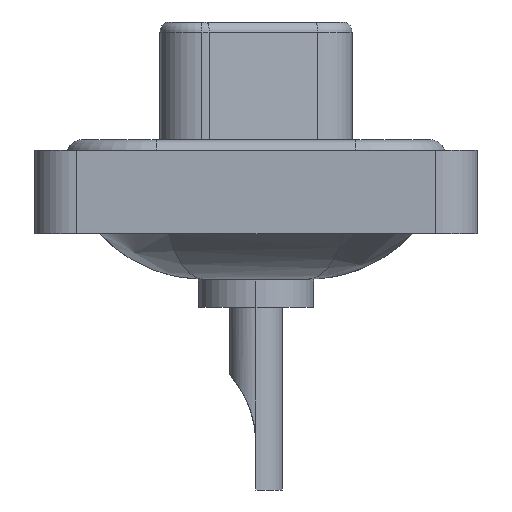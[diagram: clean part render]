
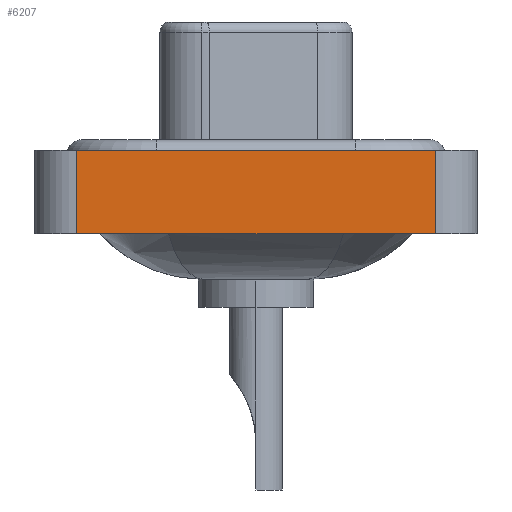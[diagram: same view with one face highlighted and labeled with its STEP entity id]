
A CAD part, left-side view. The second image highlights one B-rep face of the part: STEP entity #6207.
In plain terms, the highlighted planar face has unit normal (-1, 0, 0).
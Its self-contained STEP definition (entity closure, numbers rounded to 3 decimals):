
#63 = VECTOR ( 'NONE', #16092, 1000. ) ;
#124 = EDGE_CURVE ( 'NONE', #1892, #11301, #15623, .T. ) ;
#717 = EDGE_CURVE ( 'NONE', #1892, #13028, #8672, .T. ) ;
#1154 = CARTESIAN_POINT ( 'NONE',  ( -7.3, 8.55, -3.6 ) ) ;
#1475 = LINE ( 'NONE', #16376, #5774 ) ;
#1880 = EDGE_LOOP ( 'NONE', ( #2980, #11011, #18553, #13517 ) ) ;
#1892 = VERTEX_POINT ( 'NONE', #1154 ) ;
#2816 = CARTESIAN_POINT ( 'NONE',  ( -7.3, -8.55, 0.4 ) ) ;
#2980 = ORIENTED_EDGE ( 'NONE', *, *, #11408, .T. ) ;
#3390 = VERTEX_POINT ( 'NONE', #2816 ) ;
#4341 = LINE ( 'NONE', #8481, #63 ) ;
#5320 = CARTESIAN_POINT ( 'NONE',  ( -7.3, 8.55, 0.4 ) ) ;
#5774 = VECTOR ( 'NONE', #14998, 1000. ) ;
#6207 = ADVANCED_FACE ( 'NONE', ( #19121 ), #15877, .T. ) ;
#7223 = VECTOR ( 'NONE', #14038, 1000. ) ;
#8481 = CARTESIAN_POINT ( 'NONE',  ( -7.3, -8.55, -3.6 ) ) ;
#8672 = LINE ( 'NONE', #9965, #11480 ) ;
#9965 = CARTESIAN_POINT ( 'NONE',  ( -7.3, -8.55, -3.6 ) ) ;
#11011 = ORIENTED_EDGE ( 'NONE', *, *, #19383, .F. ) ;
#11301 = VERTEX_POINT ( 'NONE', #5320 ) ;
#11408 = EDGE_CURVE ( 'NONE', #13028, #3390, #4341, .T. ) ;
#11480 = VECTOR ( 'NONE', #14500, 1000. ) ;
#12891 = DIRECTION ( 'NONE',  ( 0., 0., 1. ) ) ;
#13028 = VERTEX_POINT ( 'NONE', #13631 ) ;
#13517 = ORIENTED_EDGE ( 'NONE', *, *, #717, .T. ) ;
#13631 = CARTESIAN_POINT ( 'NONE',  ( -7.3, -8.55, -3.6 ) ) ;
#14038 = DIRECTION ( 'NONE',  ( 0., 0., 1. ) ) ;
#14481 = CARTESIAN_POINT ( 'NONE',  ( -7.3, -8.55, -3.6 ) ) ;
#14500 = DIRECTION ( 'NONE',  ( 0., -1., 0. ) ) ;
#14998 = DIRECTION ( 'NONE',  ( 0., -1., 0. ) ) ;
#15531 = CARTESIAN_POINT ( 'NONE',  ( -7.3, 8.55, -3.6 ) ) ;
#15623 = LINE ( 'NONE', #15531, #7223 ) ;
#15772 = DIRECTION ( 'NONE',  ( -1., 0., 0. ) ) ;
#15877 = PLANE ( 'NONE',  #17560 ) ;
#16092 = DIRECTION ( 'NONE',  ( 0., 0., 1. ) ) ;
#16376 = CARTESIAN_POINT ( 'NONE',  ( -7.3, -8.55, 0.4 ) ) ;
#17560 = AXIS2_PLACEMENT_3D ( 'NONE', #14481, #15772, #12891 ) ;
#18553 = ORIENTED_EDGE ( 'NONE', *, *, #124, .F. ) ;
#19121 = FACE_OUTER_BOUND ( 'NONE', #1880, .T. ) ;
#19383 = EDGE_CURVE ( 'NONE', #11301, #3390, #1475, .T. ) ;
